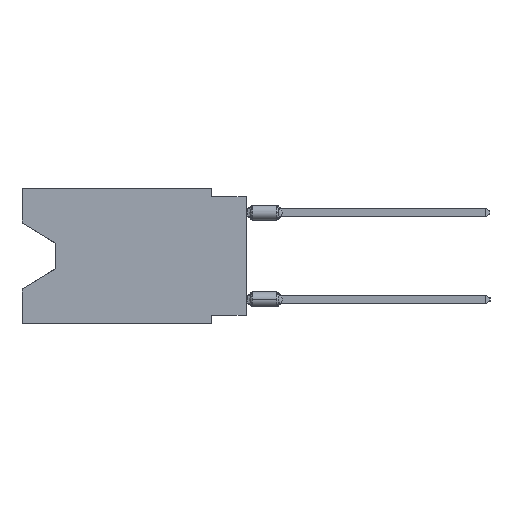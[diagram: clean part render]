
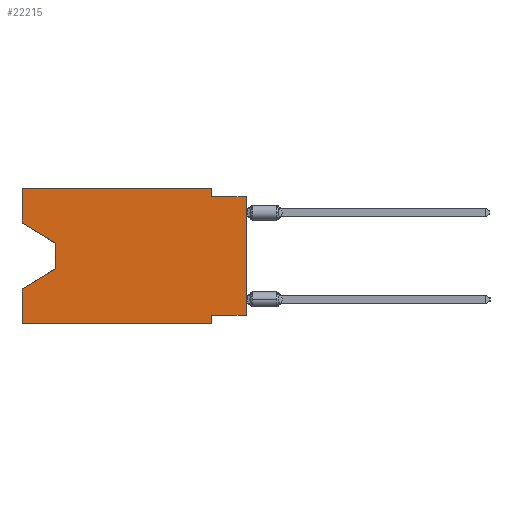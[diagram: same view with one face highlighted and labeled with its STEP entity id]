
A CAD part, left-side view. The second image highlights one B-rep face of the part: STEP entity #22215.
In plain terms, the highlighted planar face has unit normal (-1, 0, 0).
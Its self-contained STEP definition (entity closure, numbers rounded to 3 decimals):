
#1402 = ORIENTED_EDGE ( 'NONE', *, *, #40572, .F. ) ;
#2962 = CARTESIAN_POINT ( 'NONE',  ( 0., 16.383, 0. ) ) ;
#3411 = DIRECTION ( 'NONE',  ( 0., 0.855, -0.519 ) ) ;
#4029 = EDGE_CURVE ( 'NONE', #30123, #47087, #24794, .T. ) ;
#4061 = EDGE_LOOP ( 'NONE', ( #28514, #46597, #52014, #26892, #11090, #26001, #1402, #34358, #29712, #41848, #17835, #25426 ) ) ;
#4108 = FACE_OUTER_BOUND ( 'NONE', #4061, .T. ) ;
#5366 = DIRECTION ( 'NONE',  ( 0., 0., -1. ) ) ;
#5641 = LINE ( 'NONE', #19662, #11402 ) ;
#7094 = EDGE_CURVE ( 'NONE', #43811, #39300, #31482, .T. ) ;
#7530 = VECTOR ( 'NONE', #27089, 1000. ) ;
#7829 = VECTOR ( 'NONE', #3411, 1000. ) ;
#8823 = EDGE_CURVE ( 'NONE', #40262, #50683, #5641, .T. ) ;
#8929 = EDGE_CURVE ( 'NONE', #47087, #20732, #41336, .T. ) ;
#9521 = CARTESIAN_POINT ( 'NONE',  ( 0., 0., 0. ) ) ;
#11090 = ORIENTED_EDGE ( 'NONE', *, *, #31076, .T. ) ;
#11367 = VERTEX_POINT ( 'NONE', #16908 ) ;
#11402 = VECTOR ( 'NONE', #14718, 1000. ) ;
#11963 = LINE ( 'NONE', #29810, #45919 ) ;
#13334 = EDGE_CURVE ( 'NONE', #19843, #16533, #11963, .T. ) ;
#13738 = CARTESIAN_POINT ( 'NONE',  ( 0., 16.383, -2.546 ) ) ;
#13834 = EDGE_CURVE ( 'NONE', #30123, #11367, #43041, .T. ) ;
#14466 = CARTESIAN_POINT ( 'NONE',  ( 0., 2.54, 0. ) ) ;
#14718 = DIRECTION ( 'NONE',  ( 0., 0., 1. ) ) ;
#15997 = EDGE_CURVE ( 'NONE', #20732, #50683, #31494, .T. ) ;
#16016 = DIRECTION ( 'NONE',  ( 0., -0.855, -0.519 ) ) ;
#16405 = EDGE_CURVE ( 'NONE', #44087, #57688, #22918, .T. ) ;
#16533 = VERTEX_POINT ( 'NONE', #28173 ) ;
#16908 = CARTESIAN_POINT ( 'NONE',  ( 0., 16.383, 0. ) ) ;
#17835 = ORIENTED_EDGE ( 'NONE', *, *, #29217, .F. ) ;
#18240 = CARTESIAN_POINT ( 'NONE',  ( 0., 2.54, 0. ) ) ;
#18961 = VECTOR ( 'NONE', #47055, 1000. ) ;
#19096 = CARTESIAN_POINT ( 'NONE',  ( 0., 13.97, -4.013 ) ) ;
#19662 = CARTESIAN_POINT ( 'NONE',  ( 0., 16.383, 0. ) ) ;
#19843 = VERTEX_POINT ( 'NONE', #57299 ) ;
#20062 = CARTESIAN_POINT ( 'NONE',  ( 0., 16.383, -7.36 ) ) ;
#20713 = VECTOR ( 'NONE', #46287, 1000. ) ;
#20732 = VERTEX_POINT ( 'NONE', #40443 ) ;
#20996 = VECTOR ( 'NONE', #41936, 1000. ) ;
#22215 = ADVANCED_FACE ( 'NONE', ( #4108 ), #57652, .F. ) ;
#22420 = CARTESIAN_POINT ( 'NONE',  ( 0., 0., -9.271 ) ) ;
#22918 = LINE ( 'NONE', #18240, #47225 ) ;
#24661 = CARTESIAN_POINT ( 'NONE',  ( 0., 0., -0.635 ) ) ;
#24671 = LINE ( 'NONE', #45756, #20996 ) ;
#24794 = LINE ( 'NONE', #28911, #25045 ) ;
#25045 = VECTOR ( 'NONE', #16016, 1000. ) ;
#25426 = ORIENTED_EDGE ( 'NONE', *, *, #13834, .F. ) ;
#26001 = ORIENTED_EDGE ( 'NONE', *, *, #13334, .F. ) ;
#26815 = CARTESIAN_POINT ( 'NONE',  ( 0., 13.97, -5.893 ) ) ;
#26892 = ORIENTED_EDGE ( 'NONE', *, *, #8823, .F. ) ;
#27089 = DIRECTION ( 'NONE',  ( 0., 0., 1. ) ) ;
#27877 = CARTESIAN_POINT ( 'NONE',  ( 0., 0., -0.635 ) ) ;
#28173 = CARTESIAN_POINT ( 'NONE',  ( 0., 2.54, -9.906 ) ) ;
#28514 = ORIENTED_EDGE ( 'NONE', *, *, #4029, .T. ) ;
#28547 = VECTOR ( 'NONE', #49057, 1000. ) ;
#28911 = CARTESIAN_POINT ( 'NONE',  ( 0., 16.383, -2.546 ) ) ;
#29217 = EDGE_CURVE ( 'NONE', #11367, #44087, #29897, .T. ) ;
#29634 = LINE ( 'NONE', #24661, #43765 ) ;
#29712 = ORIENTED_EDGE ( 'NONE', *, *, #53757, .F. ) ;
#29810 = CARTESIAN_POINT ( 'NONE',  ( 0., 2.54, -9.906 ) ) ;
#29897 = LINE ( 'NONE', #35448, #18961 ) ;
#30123 = VERTEX_POINT ( 'NONE', #13738 ) ;
#31028 = CARTESIAN_POINT ( 'NONE',  ( 0., 16.383, 0. ) ) ;
#31076 = EDGE_CURVE ( 'NONE', #40262, #16533, #24671, .T. ) ;
#31482 = LINE ( 'NONE', #9521, #7530 ) ;
#31494 = LINE ( 'NONE', #26815, #7829 ) ;
#32178 = CARTESIAN_POINT ( 'NONE',  ( 0., 2.54, -0.635 ) ) ;
#33734 = DIRECTION ( 'NONE',  ( 0., -1., 0. ) ) ;
#34358 = ORIENTED_EDGE ( 'NONE', *, *, #7094, .T. ) ;
#35448 = CARTESIAN_POINT ( 'NONE',  ( 0., 16.383, 0. ) ) ;
#36331 = AXIS2_PLACEMENT_3D ( 'NONE', #31028, #48873, #36548 ) ;
#36548 = DIRECTION ( 'NONE',  ( 0., 0., -1. ) ) ;
#38186 = CARTESIAN_POINT ( 'NONE',  ( 0., 0., -9.271 ) ) ;
#39300 = VERTEX_POINT ( 'NONE', #27877 ) ;
#40262 = VERTEX_POINT ( 'NONE', #55239 ) ;
#40443 = CARTESIAN_POINT ( 'NONE',  ( 0., 13.97, -5.893 ) ) ;
#40572 = EDGE_CURVE ( 'NONE', #43811, #19843, #44663, .T. ) ;
#41336 = LINE ( 'NONE', #19096, #20713 ) ;
#41848 = ORIENTED_EDGE ( 'NONE', *, *, #16405, .F. ) ;
#41936 = DIRECTION ( 'NONE',  ( 0., -1., 0. ) ) ;
#43041 = LINE ( 'NONE', #2962, #44134 ) ;
#43765 = VECTOR ( 'NONE', #33734, 1000. ) ;
#43811 = VERTEX_POINT ( 'NONE', #38186 ) ;
#44087 = VERTEX_POINT ( 'NONE', #14466 ) ;
#44134 = VECTOR ( 'NONE', #56513, 1000. ) ;
#44663 = LINE ( 'NONE', #22420, #28547 ) ;
#45756 = CARTESIAN_POINT ( 'NONE',  ( 0., 16.383, -9.906 ) ) ;
#45919 = VECTOR ( 'NONE', #47653, 1000. ) ;
#46287 = DIRECTION ( 'NONE',  ( 0., 0., -1. ) ) ;
#46597 = ORIENTED_EDGE ( 'NONE', *, *, #8929, .T. ) ;
#47055 = DIRECTION ( 'NONE',  ( 0., -1., 0. ) ) ;
#47087 = VERTEX_POINT ( 'NONE', #54116 ) ;
#47225 = VECTOR ( 'NONE', #5366, 1000. ) ;
#47653 = DIRECTION ( 'NONE',  ( 0., 0., -1. ) ) ;
#48873 = DIRECTION ( 'NONE',  ( 1., 0., 0. ) ) ;
#49057 = DIRECTION ( 'NONE',  ( 0., 1., 0. ) ) ;
#50683 = VERTEX_POINT ( 'NONE', #20062 ) ;
#52014 = ORIENTED_EDGE ( 'NONE', *, *, #15997, .T. ) ;
#53757 = EDGE_CURVE ( 'NONE', #57688, #39300, #29634, .T. ) ;
#54116 = CARTESIAN_POINT ( 'NONE',  ( 0., 13.97, -4.013 ) ) ;
#55239 = CARTESIAN_POINT ( 'NONE',  ( 0., 16.383, -9.906 ) ) ;
#56513 = DIRECTION ( 'NONE',  ( 0., 0., 1. ) ) ;
#57299 = CARTESIAN_POINT ( 'NONE',  ( 0., 2.54, -9.271 ) ) ;
#57652 = PLANE ( 'NONE',  #36331 ) ;
#57688 = VERTEX_POINT ( 'NONE', #32178 ) ;
